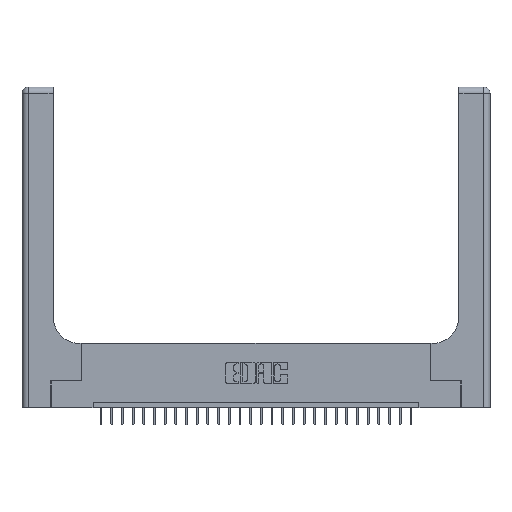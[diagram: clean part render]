
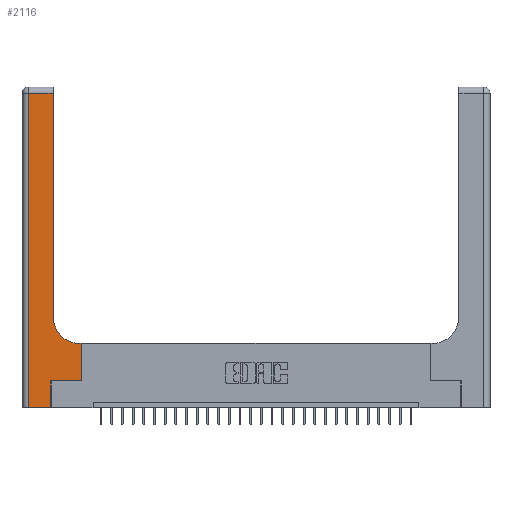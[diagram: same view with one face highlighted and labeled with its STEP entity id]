
A CAD part, top view. The second image highlights one B-rep face of the part: STEP entity #2116.
In plain terms, the highlighted planar face has unit normal (0, 0, 1).
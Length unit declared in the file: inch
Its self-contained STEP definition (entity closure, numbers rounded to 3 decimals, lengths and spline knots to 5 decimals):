
#6 = EDGE_CURVE ( 'NONE', #5424, #12609, #3491, .T. ) ;
#422 = VERTEX_POINT ( 'NONE', #28064 ) ;
#867 = CARTESIAN_POINT ( 'NONE',  ( 0.269, 0., 0.37 ) ) ;
#1100 = CARTESIAN_POINT ( 'NONE',  ( 0.5585, 0.6, 0.37 ) ) ;
#2116 = ADVANCED_FACE ( 'NONE', ( #27694 ), #3154, .F. ) ;
#2942 = CARTESIAN_POINT ( 'NONE',  ( 0.2915, 2.94, 0.37 ) ) ;
#3154 = PLANE ( 'NONE',  #6972 ) ;
#3491 = LINE ( 'NONE', #14748, #20946 ) ;
#5138 = CARTESIAN_POINT ( 'NONE',  ( 0.269, 0., 0.37 ) ) ;
#5424 = VERTEX_POINT ( 'NONE', #21315 ) ;
#5484 = ORIENTED_EDGE ( 'NONE', *, *, #6102, .T. ) ;
#6102 = EDGE_CURVE ( 'NONE', #13223, #10404, #6493, .T. ) ;
#6493 = LINE ( 'NONE', #26647, #11845 ) ;
#6624 = LINE ( 'NONE', #20515, #15851 ) ;
#6718 = ORIENTED_EDGE ( 'NONE', *, *, #8543, .T. ) ;
#6972 = AXIS2_PLACEMENT_3D ( 'NONE', #19168, #7612, #8010 ) ;
#7612 = DIRECTION ( 'NONE',  ( 0., 0., -1. ) ) ;
#7819 = DIRECTION ( 'NONE',  ( 0., 1., 0. ) ) ;
#8010 = DIRECTION ( 'NONE',  ( -1., 0., 0. ) ) ;
#8543 = EDGE_CURVE ( 'NONE', #17578, #5424, #27462, .T. ) ;
#8592 = DIRECTION ( 'NONE',  ( -1., 0., 0. ) ) ;
#8625 = VECTOR ( 'NONE', #7819, 39.37008 ) ;
#8741 = CARTESIAN_POINT ( 'NONE',  ( 0.06, 3., 0.37 ) ) ;
#8841 = DIRECTION ( 'NONE',  ( 0., -1., 0. ) ) ;
#8874 = ORIENTED_EDGE ( 'NONE', *, *, #17436, .T. ) ;
#9651 = ORIENTED_EDGE ( 'NONE', *, *, #9770, .T. ) ;
#9770 = EDGE_CURVE ( 'NONE', #10404, #12678, #17392, .T. ) ;
#9887 = EDGE_CURVE ( 'NONE', #16589, #422, #28083, .T. ) ;
#10404 = VERTEX_POINT ( 'NONE', #17344 ) ;
#10714 = VECTOR ( 'NONE', #10868, 39.37008 ) ;
#10868 = DIRECTION ( 'NONE',  ( 0., 1., 0. ) ) ;
#11413 = EDGE_CURVE ( 'NONE', #12678, #27264, #6624, .T. ) ;
#11464 = DIRECTION ( 'NONE',  ( 0., 1., 0. ) ) ;
#11845 = VECTOR ( 'NONE', #17363, 39.37008 ) ;
#11915 = CARTESIAN_POINT ( 'NONE',  ( 0.2915, 0.85, 0.37 ) ) ;
#12102 = CARTESIAN_POINT ( 'NONE',  ( 0., 0., 0.37 ) ) ;
#12197 = VECTOR ( 'NONE', #14341, 39.37008 ) ;
#12609 = VERTEX_POINT ( 'NONE', #26582 ) ;
#12678 = VERTEX_POINT ( 'NONE', #11915 ) ;
#12810 = ORIENTED_EDGE ( 'NONE', *, *, #6, .T. ) ;
#13158 = CARTESIAN_POINT ( 'NONE',  ( 0.06, 2.94, 0.37 ) ) ;
#13223 = VERTEX_POINT ( 'NONE', #1100 ) ;
#14341 = DIRECTION ( 'NONE',  ( 1., 0., 0. ) ) ;
#14748 = CARTESIAN_POINT ( 'NONE',  ( 0.269, 0.25, 0.37 ) ) ;
#15257 = EDGE_LOOP ( 'NONE', ( #22994, #22701, #17997, #17329, #6718, #12810, #8874, #5484, #9651 ) ) ;
#15653 = CARTESIAN_POINT ( 'NONE',  ( 0.5415, 0.85, 0.37 ) ) ;
#15851 = VECTOR ( 'NONE', #11464, 39.37008 ) ;
#16380 = EDGE_CURVE ( 'NONE', #422, #17578, #28911, .T. ) ;
#16589 = VERTEX_POINT ( 'NONE', #13158 ) ;
#17210 = AXIS2_PLACEMENT_3D ( 'NONE', #15653, #29310, #26853 ) ;
#17329 = ORIENTED_EDGE ( 'NONE', *, *, #16380, .T. ) ;
#17344 = CARTESIAN_POINT ( 'NONE',  ( 0.5415, 0.6, 0.37 ) ) ;
#17363 = DIRECTION ( 'NONE',  ( -1., 0., 0. ) ) ;
#17392 = CIRCLE ( 'NONE', #17210, 0.25 ) ;
#17395 = EDGE_CURVE ( 'NONE', #27264, #16589, #24606, .T. ) ;
#17436 = EDGE_CURVE ( 'NONE', #12609, #13223, #17815, .T. ) ;
#17578 = VERTEX_POINT ( 'NONE', #5138 ) ;
#17707 = CARTESIAN_POINT ( 'NONE',  ( 0.5585, 0.25, 0.37 ) ) ;
#17815 = LINE ( 'NONE', #17707, #10714 ) ;
#17997 = ORIENTED_EDGE ( 'NONE', *, *, #9887, .T. ) ;
#19168 = CARTESIAN_POINT ( 'NONE',  ( 0., 3., 0.37 ) ) ;
#20271 = VECTOR ( 'NONE', #8841, 39.37008 ) ;
#20515 = CARTESIAN_POINT ( 'NONE',  ( 0.2915, 3., 0.37 ) ) ;
#20946 = VECTOR ( 'NONE', #26323, 39.37008 ) ;
#21315 = CARTESIAN_POINT ( 'NONE',  ( 0.269, 0.25, 0.37 ) ) ;
#22701 = ORIENTED_EDGE ( 'NONE', *, *, #17395, .T. ) ;
#22994 = ORIENTED_EDGE ( 'NONE', *, *, #11413, .T. ) ;
#23156 = VECTOR ( 'NONE', #8592, 39.37008 ) ;
#24504 = CARTESIAN_POINT ( 'NONE',  ( 0., 2.94, 0.37 ) ) ;
#24606 = LINE ( 'NONE', #24504, #23156 ) ;
#26323 = DIRECTION ( 'NONE',  ( 1., 0., 0. ) ) ;
#26582 = CARTESIAN_POINT ( 'NONE',  ( 0.5585, 0.25, 0.37 ) ) ;
#26647 = CARTESIAN_POINT ( 'NONE',  ( 0.2915, 0.6, 0.37 ) ) ;
#26853 = DIRECTION ( 'NONE',  ( 1., 0., 0. ) ) ;
#27264 = VERTEX_POINT ( 'NONE', #2942 ) ;
#27462 = LINE ( 'NONE', #867, #8625 ) ;
#27694 = FACE_OUTER_BOUND ( 'NONE', #15257, .T. ) ;
#28064 = CARTESIAN_POINT ( 'NONE',  ( 0.06, 0., 0.37 ) ) ;
#28083 = LINE ( 'NONE', #8741, #20271 ) ;
#28911 = LINE ( 'NONE', #12102, #12197 ) ;
#29310 = DIRECTION ( 'NONE',  ( 0., 0., -1. ) ) ;
